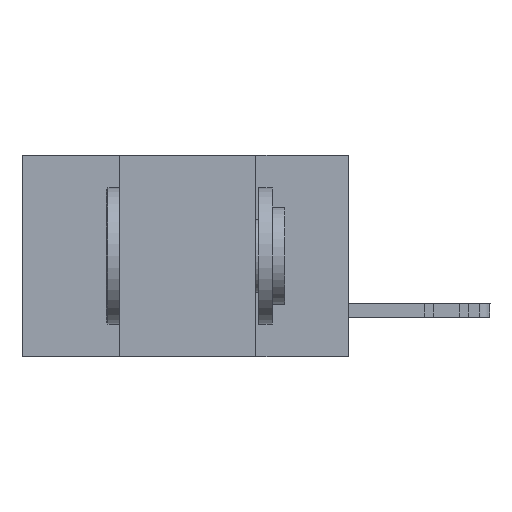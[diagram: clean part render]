
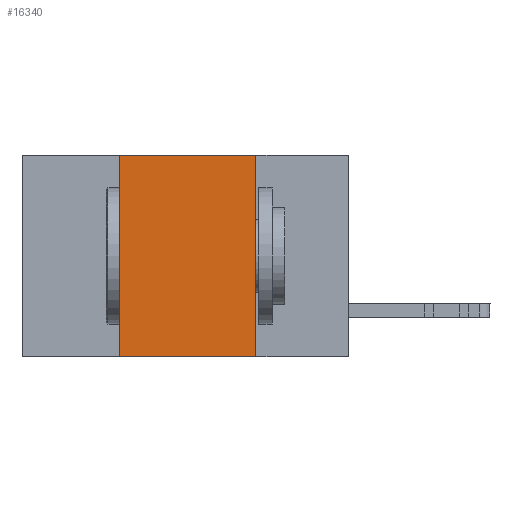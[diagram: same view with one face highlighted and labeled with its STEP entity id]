
A CAD part, left-side view. The second image highlights one B-rep face of the part: STEP entity #16340.
In plain terms, the highlighted planar face has unit normal (-1, 0, 0).
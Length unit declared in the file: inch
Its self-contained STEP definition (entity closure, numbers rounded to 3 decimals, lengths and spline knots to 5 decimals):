
#1787 = DIRECTION ( 'NONE',  ( 0., -1., 0. ) ) ;
#1861 = CARTESIAN_POINT ( 'NONE',  ( 0., 0.6, -0.37 ) ) ;
#2212 = CARTESIAN_POINT ( 'NONE',  ( 0., 0.17, -0.37 ) ) ;
#2744 = VERTEX_POINT ( 'NONE', #5608 ) ;
#2899 = VECTOR ( 'NONE', #4274, 39.37008 ) ;
#3123 = CARTESIAN_POINT ( 'NONE',  ( 0., 0.42, 0. ) ) ;
#4220 = CARTESIAN_POINT ( 'NONE',  ( 0., 0.42, -0.37 ) ) ;
#4274 = DIRECTION ( 'NONE',  ( 0., 0., 1. ) ) ;
#5516 = EDGE_CURVE ( 'NONE', #14192, #15702, #16807, .T. ) ;
#5551 = ORIENTED_EDGE ( 'NONE', *, *, #15268, .F. ) ;
#5608 = CARTESIAN_POINT ( 'NONE',  ( 0., 0.42, -0.37 ) ) ;
#6570 = EDGE_LOOP ( 'NONE', ( #13764, #19815, #5551, #11119 ) ) ;
#7018 = FACE_OUTER_BOUND ( 'NONE', #6570, .T. ) ;
#10824 = EDGE_CURVE ( 'NONE', #15702, #17331, #19697, .T. ) ;
#11119 = ORIENTED_EDGE ( 'NONE', *, *, #14323, .T. ) ;
#12314 = DIRECTION ( 'NONE',  ( 0., 0., -1. ) ) ;
#12791 = CARTESIAN_POINT ( 'NONE',  ( 0., 0.17, -0.37 ) ) ;
#13764 = ORIENTED_EDGE ( 'NONE', *, *, #10824, .F. ) ;
#13885 = DIRECTION ( 'NONE',  ( 0., 0., -1. ) ) ;
#13917 = DIRECTION ( 'NONE',  ( 1., 0., 0. ) ) ;
#13920 = CARTESIAN_POINT ( 'NONE',  ( 0., 0.6, 0. ) ) ;
#13943 = PLANE ( 'NONE',  #17334 ) ;
#14184 = LINE ( 'NONE', #1861, #23237 ) ;
#14192 = VERTEX_POINT ( 'NONE', #3123 ) ;
#14323 = EDGE_CURVE ( 'NONE', #2744, #17331, #14184, .T. ) ;
#15268 = EDGE_CURVE ( 'NONE', #2744, #14192, #22119, .T. ) ;
#15702 = VERTEX_POINT ( 'NONE', #20725 ) ;
#16340 = ADVANCED_FACE ( 'NONE', ( #7018 ), #13943, .F. ) ;
#16807 = LINE ( 'NONE', #19486, #22729 ) ;
#17331 = VERTEX_POINT ( 'NONE', #2212 ) ;
#17334 = AXIS2_PLACEMENT_3D ( 'NONE', #13920, #13917, #13885 ) ;
#19328 = DIRECTION ( 'NONE',  ( 0., -1., 0. ) ) ;
#19486 = CARTESIAN_POINT ( 'NONE',  ( 0., 0.6, 0. ) ) ;
#19697 = LINE ( 'NONE', #12791, #20279 ) ;
#19815 = ORIENTED_EDGE ( 'NONE', *, *, #5516, .F. ) ;
#20279 = VECTOR ( 'NONE', #12314, 39.37008 ) ;
#20725 = CARTESIAN_POINT ( 'NONE',  ( 0., 0.17, 0. ) ) ;
#22119 = LINE ( 'NONE', #4220, #2899 ) ;
#22729 = VECTOR ( 'NONE', #19328, 39.37008 ) ;
#23237 = VECTOR ( 'NONE', #1787, 39.37008 ) ;
